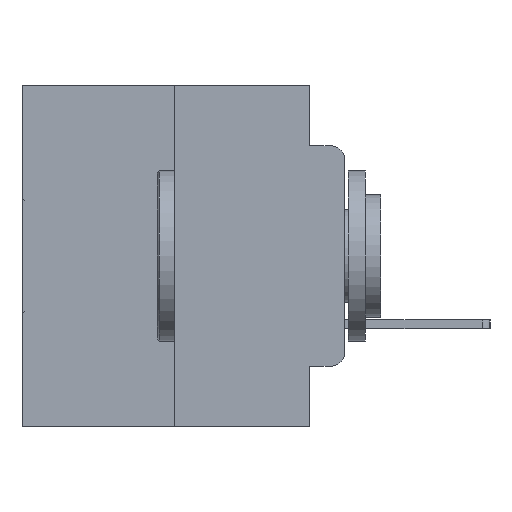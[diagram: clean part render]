
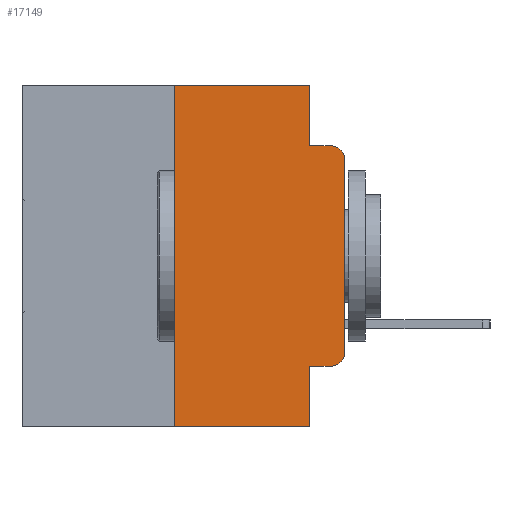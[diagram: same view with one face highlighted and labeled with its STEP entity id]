
A CAD part, left-side view. The second image highlights one B-rep face of the part: STEP entity #17149.
In plain terms, the highlighted planar face has unit normal (-1, 0, 0).
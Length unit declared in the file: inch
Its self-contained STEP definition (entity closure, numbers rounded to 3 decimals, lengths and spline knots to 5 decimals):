
#51 = VECTOR ( 'NONE', #497, 39.37008 ) ;
#497 = DIRECTION ( 'NONE',  ( 0., 0., 1. ) ) ;
#1078 = ORIENTED_EDGE ( 'NONE', *, *, #2065, .F. ) ;
#1616 = EDGE_LOOP ( 'NONE', ( #14568, #29358, #1078, #22708, #5870, #26937, #16380, #19206, #19901, #11347 ) ) ;
#2065 = EDGE_CURVE ( 'NONE', #5038, #2870, #14802, .T. ) ;
#2096 = VECTOR ( 'NONE', #25385, 39.37008 ) ;
#2870 = VERTEX_POINT ( 'NONE', #14580 ) ;
#3049 = VERTEX_POINT ( 'NONE', #9008 ) ;
#3101 = VERTEX_POINT ( 'NONE', #20416 ) ;
#3308 = EDGE_CURVE ( 'NONE', #21781, #14573, #17240, .T. ) ;
#3548 = LINE ( 'NONE', #14119, #2096 ) ;
#3964 = LINE ( 'NONE', #6939, #27569 ) ;
#4961 = VECTOR ( 'NONE', #16900, 39.37008 ) ;
#4986 = EDGE_CURVE ( 'NONE', #13604, #13702, #19952, .T. ) ;
#5038 = VERTEX_POINT ( 'NONE', #22105 ) ;
#5405 = CARTESIAN_POINT ( 'NONE',  ( 0., 0.02, -0.3915 ) ) ;
#5492 = VECTOR ( 'NONE', #8560, 39.37008 ) ;
#5860 = DIRECTION ( 'NONE',  ( 0., 0., -1. ) ) ;
#5870 = ORIENTED_EDGE ( 'NONE', *, *, #3308, .F. ) ;
#6939 = CARTESIAN_POINT ( 'NONE',  ( 0., 0.051, -0.4115 ) ) ;
#7583 = DIRECTION ( 'NONE',  ( -1., 0., 0. ) ) ;
#7739 = DIRECTION ( 'NONE',  ( 0., 0., -1. ) ) ;
#8560 = DIRECTION ( 'NONE',  ( 0., 0., 1. ) ) ;
#8577 = EDGE_CURVE ( 'NONE', #26242, #3049, #28629, .T. ) ;
#8951 = CARTESIAN_POINT ( 'NONE',  ( 0., 0.02, -0.4115 ) ) ;
#9008 = CARTESIAN_POINT ( 'NONE',  ( 0., 0., -0.3915 ) ) ;
#9212 = CARTESIAN_POINT ( 'NONE',  ( 0., 0.25, 0. ) ) ;
#11347 = ORIENTED_EDGE ( 'NONE', *, *, #8577, .T. ) ;
#11931 = FACE_OUTER_BOUND ( 'NONE', #1616, .T. ) ;
#12388 = DIRECTION ( 'NONE',  ( 0., 0., -1. ) ) ;
#12804 = VERTEX_POINT ( 'NONE', #27446 ) ;
#13374 = AXIS2_PLACEMENT_3D ( 'NONE', #21319, #7583, #23568 ) ;
#13604 = VERTEX_POINT ( 'NONE', #23999 ) ;
#13702 = VERTEX_POINT ( 'NONE', #19920 ) ;
#13922 = DIRECTION ( 'NONE',  ( 0., 0., -1. ) ) ;
#14119 = CARTESIAN_POINT ( 'NONE',  ( 0., 0.473, -0.5 ) ) ;
#14568 = ORIENTED_EDGE ( 'NONE', *, *, #25840, .T. ) ;
#14573 = VERTEX_POINT ( 'NONE', #27165 ) ;
#14580 = CARTESIAN_POINT ( 'NONE',  ( 0., 0.02, -0.0885 ) ) ;
#14802 = LINE ( 'NONE', #21689, #26091 ) ;
#15426 = EDGE_CURVE ( 'NONE', #13604, #26242, #3964, .T. ) ;
#15638 = EDGE_CURVE ( 'NONE', #14573, #5038, #16642, .T. ) ;
#15933 = VECTOR ( 'NONE', #12388, 39.37008 ) ;
#16173 = DIRECTION ( 'NONE',  ( 0., -1., 0. ) ) ;
#16380 = ORIENTED_EDGE ( 'NONE', *, *, #20905, .T. ) ;
#16642 = LINE ( 'NONE', #17003, #15933 ) ;
#16900 = DIRECTION ( 'NONE',  ( 0., -1., 0. ) ) ;
#17003 = CARTESIAN_POINT ( 'NONE',  ( 0., 0.051, 0. ) ) ;
#17114 = CARTESIAN_POINT ( 'NONE',  ( 0., 0.473, 0. ) ) ;
#17149 = ADVANCED_FACE ( 'NONE', ( #11931 ), #20680, .F. ) ;
#17240 = LINE ( 'NONE', #17114, #4961 ) ;
#18316 = CARTESIAN_POINT ( 'NONE',  ( 0., 0.473, 0. ) ) ;
#18462 = AXIS2_PLACEMENT_3D ( 'NONE', #5405, #21470, #7739 ) ;
#18544 = LINE ( 'NONE', #27966, #51 ) ;
#19206 = ORIENTED_EDGE ( 'NONE', *, *, #4986, .F. ) ;
#19901 = ORIENTED_EDGE ( 'NONE', *, *, #15426, .T. ) ;
#19920 = CARTESIAN_POINT ( 'NONE',  ( 0., 0.051, -0.5 ) ) ;
#19952 = LINE ( 'NONE', #21913, #26648 ) ;
#20416 = CARTESIAN_POINT ( 'NONE',  ( 0., 0.25, -0.5 ) ) ;
#20680 = PLANE ( 'NONE',  #29031 ) ;
#20905 = EDGE_CURVE ( 'NONE', #3101, #13702, #3548, .T. ) ;
#21319 = CARTESIAN_POINT ( 'NONE',  ( 0., 0.02, -0.1085 ) ) ;
#21470 = DIRECTION ( 'NONE',  ( -1., 0., 0. ) ) ;
#21689 = CARTESIAN_POINT ( 'NONE',  ( 0., 0.051, -0.0885 ) ) ;
#21781 = VERTEX_POINT ( 'NONE', #9212 ) ;
#21913 = CARTESIAN_POINT ( 'NONE',  ( 0., 0.051, 0. ) ) ;
#22105 = CARTESIAN_POINT ( 'NONE',  ( 0., 0.051, -0.0885 ) ) ;
#22708 = ORIENTED_EDGE ( 'NONE', *, *, #15638, .F. ) ;
#23049 = LINE ( 'NONE', #24522, #5492 ) ;
#23568 = DIRECTION ( 'NONE',  ( 0., 0., -1. ) ) ;
#23999 = CARTESIAN_POINT ( 'NONE',  ( 0., 0.051, -0.4115 ) ) ;
#24522 = CARTESIAN_POINT ( 'NONE',  ( 0., 0.25, 0. ) ) ;
#25385 = DIRECTION ( 'NONE',  ( 0., -1., 0. ) ) ;
#25840 = EDGE_CURVE ( 'NONE', #3049, #12804, #18544, .T. ) ;
#26091 = VECTOR ( 'NONE', #16173, 39.37008 ) ;
#26242 = VERTEX_POINT ( 'NONE', #8951 ) ;
#26648 = VECTOR ( 'NONE', #5860, 39.37008 ) ;
#26937 = ORIENTED_EDGE ( 'NONE', *, *, #27169, .F. ) ;
#27164 = CIRCLE ( 'NONE', #13374, 0.02 ) ;
#27165 = CARTESIAN_POINT ( 'NONE',  ( 0., 0.051, 0. ) ) ;
#27169 = EDGE_CURVE ( 'NONE', #3101, #21781, #23049, .T. ) ;
#27438 = DIRECTION ( 'NONE',  ( 0., -1., 0. ) ) ;
#27445 = DIRECTION ( 'NONE',  ( 1., 0., 0. ) ) ;
#27446 = CARTESIAN_POINT ( 'NONE',  ( 0., 0., -0.1085 ) ) ;
#27569 = VECTOR ( 'NONE', #27438, 39.37008 ) ;
#27966 = CARTESIAN_POINT ( 'NONE',  ( 0., 0., 0. ) ) ;
#28629 = CIRCLE ( 'NONE', #18462, 0.02 ) ;
#29031 = AXIS2_PLACEMENT_3D ( 'NONE', #18316, #27445, #13922 ) ;
#29358 = ORIENTED_EDGE ( 'NONE', *, *, #29382, .T. ) ;
#29382 = EDGE_CURVE ( 'NONE', #12804, #2870, #27164, .T. ) ;
